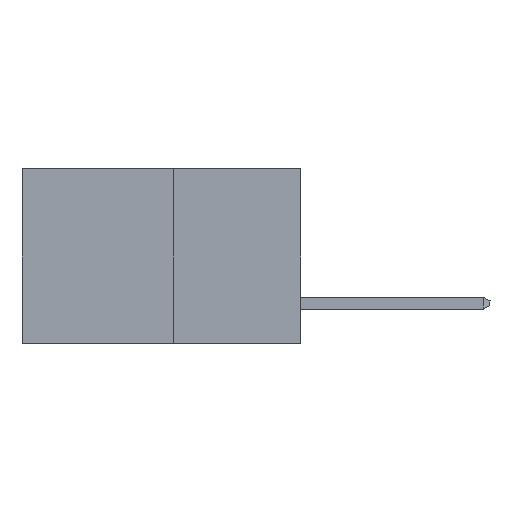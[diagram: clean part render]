
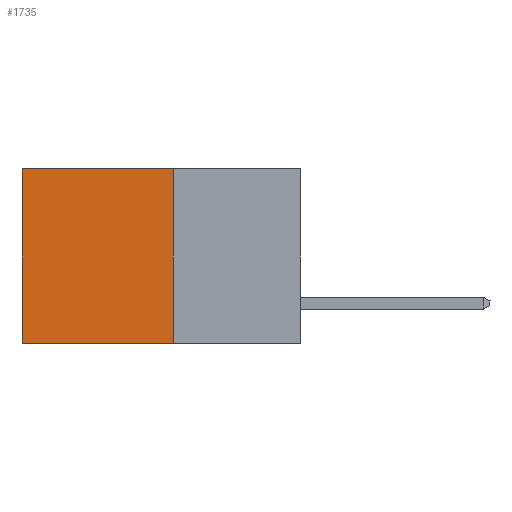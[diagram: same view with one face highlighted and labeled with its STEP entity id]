
A CAD part, left-side view. The second image highlights one B-rep face of the part: STEP entity #1735.
In plain terms, the highlighted planar face has unit normal (-1, 0, 0).
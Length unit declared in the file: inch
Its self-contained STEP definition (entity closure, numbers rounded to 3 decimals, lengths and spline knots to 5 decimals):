
#1 = DIRECTION ( 'NONE',  ( 0., 1., 0. ) ) ;
#481 = EDGE_CURVE ( 'NONE', #4050, #4359, #1978, .T. ) ;
#1171 = CARTESIAN_POINT ( 'NONE',  ( 0.277, 0.27, -0.37 ) ) ;
#1567 = ORIENTED_EDGE ( 'NONE', *, *, #8580, .F. ) ;
#1735 = ADVANCED_FACE ( 'NONE', ( #11329 ), #11409, .F. ) ;
#1908 = VECTOR ( 'NONE', #1, 39.37008 ) ;
#1978 = LINE ( 'NONE', #4585, #8972 ) ;
#2408 = LINE ( 'NONE', #8674, #4783 ) ;
#2612 = AXIS2_PLACEMENT_3D ( 'NONE', #7128, #7072, #6983 ) ;
#2710 = EDGE_CURVE ( 'NONE', #7862, #9391, #4303, .T. ) ;
#3209 = CARTESIAN_POINT ( 'NONE',  ( 0.277, 0.27, 0. ) ) ;
#4038 = ORIENTED_EDGE ( 'NONE', *, *, #2710, .F. ) ;
#4050 = VERTEX_POINT ( 'NONE', #6905 ) ;
#4303 = LINE ( 'NONE', #10856, #10790 ) ;
#4359 = VERTEX_POINT ( 'NONE', #11435 ) ;
#4585 = CARTESIAN_POINT ( 'NONE',  ( 0.277, 0.59, -0.37 ) ) ;
#4783 = VECTOR ( 'NONE', #5751, 39.37008 ) ;
#5751 = DIRECTION ( 'NONE',  ( 0., 1., 0. ) ) ;
#6174 = DIRECTION ( 'NONE',  ( 0., 0., -1. ) ) ;
#6368 = EDGE_CURVE ( 'NONE', #7862, #4050, #2408, .T. ) ;
#6905 = CARTESIAN_POINT ( 'NONE',  ( 0.277, 0.59, 0. ) ) ;
#6983 = DIRECTION ( 'NONE',  ( 0., 0., -1. ) ) ;
#7072 = DIRECTION ( 'NONE',  ( 1., 0., 0. ) ) ;
#7128 = CARTESIAN_POINT ( 'NONE',  ( 0.277, 0.27, -0.37 ) ) ;
#7633 = DIRECTION ( 'NONE',  ( 0., 0., -1. ) ) ;
#7652 = CARTESIAN_POINT ( 'NONE',  ( 0.277, 0.27, -0.37 ) ) ;
#7862 = VERTEX_POINT ( 'NONE', #3209 ) ;
#8580 = EDGE_CURVE ( 'NONE', #9391, #4359, #9226, .T. ) ;
#8674 = CARTESIAN_POINT ( 'NONE',  ( 0.277, 0.27, 0. ) ) ;
#8904 = ORIENTED_EDGE ( 'NONE', *, *, #6368, .T. ) ;
#8972 = VECTOR ( 'NONE', #6174, 39.37008 ) ;
#9226 = LINE ( 'NONE', #1171, #1908 ) ;
#9391 = VERTEX_POINT ( 'NONE', #7652 ) ;
#10790 = VECTOR ( 'NONE', #7633, 39.37008 ) ;
#10856 = CARTESIAN_POINT ( 'NONE',  ( 0.277, 0.27, -0.37 ) ) ;
#10889 = EDGE_LOOP ( 'NONE', ( #11045, #1567, #4038, #8904 ) ) ;
#11045 = ORIENTED_EDGE ( 'NONE', *, *, #481, .T. ) ;
#11329 = FACE_OUTER_BOUND ( 'NONE', #10889, .T. ) ;
#11409 = PLANE ( 'NONE',  #2612 ) ;
#11435 = CARTESIAN_POINT ( 'NONE',  ( 0.277, 0.59, -0.37 ) ) ;
